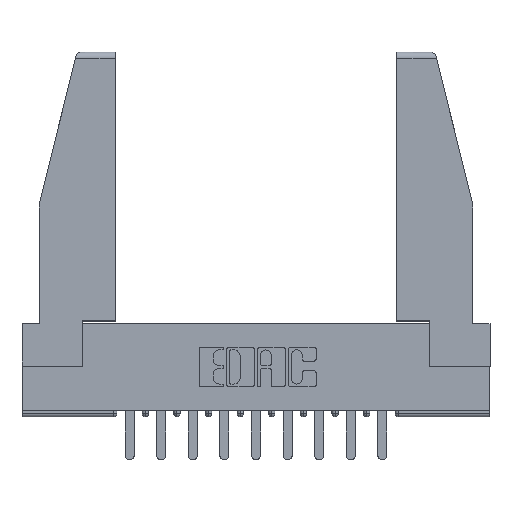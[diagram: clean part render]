
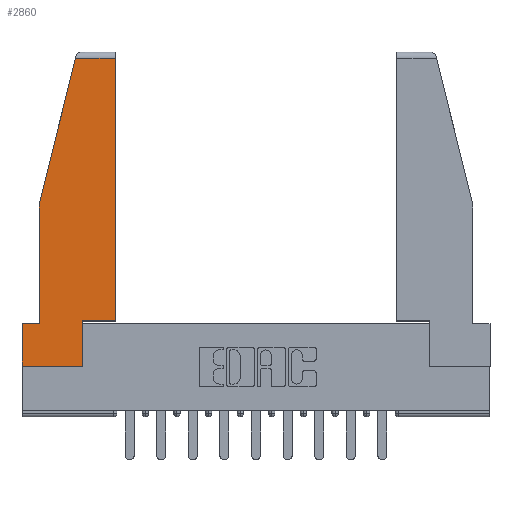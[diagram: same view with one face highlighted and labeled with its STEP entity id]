
A CAD part, top view. The second image highlights one B-rep face of the part: STEP entity #2860.
In plain terms, the highlighted planar face has unit normal (0, 0, 1).
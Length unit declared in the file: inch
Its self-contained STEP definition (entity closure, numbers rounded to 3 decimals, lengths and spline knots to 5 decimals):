
#167 = CARTESIAN_POINT ( 'NONE',  ( 0.297, 0., 0. ) ) ;
#615 = CARTESIAN_POINT ( 'NONE',  ( 0., 0., 0. ) ) ;
#668 = VECTOR ( 'NONE', #8872, 39.37008 ) ;
#1336 = ORIENTED_EDGE ( 'NONE', *, *, #2881, .T. ) ;
#1366 = VERTEX_POINT ( 'NONE', #615 ) ;
#1624 = CARTESIAN_POINT ( 'NONE',  ( 0.297, 0.223, 0. ) ) ;
#1625 = DIRECTION ( 'NONE',  ( -0.239, -0.971, 0. ) ) ;
#1884 = CARTESIAN_POINT ( 'NONE',  ( 0.461, 1.52, 0. ) ) ;
#2151 = ORIENTED_EDGE ( 'NONE', *, *, #11535, .T. ) ;
#2159 = VERTEX_POINT ( 'NONE', #7401 ) ;
#2522 = DIRECTION ( 'NONE',  ( 0., 1., 0. ) ) ;
#2757 = LINE ( 'NONE', #7891, #9374 ) ;
#2848 = VERTEX_POINT ( 'NONE', #7024 ) ;
#2860 = ADVANCED_FACE ( 'NONE', ( #3375 ), #5828, .T. ) ;
#2881 = EDGE_CURVE ( 'NONE', #3419, #1366, #15807, .T. ) ;
#2916 = VECTOR ( 'NONE', #1625, 39.37008 ) ;
#3042 = ORIENTED_EDGE ( 'NONE', *, *, #3431, .T. ) ;
#3375 = FACE_OUTER_BOUND ( 'NONE', #16056, .T. ) ;
#3419 = VERTEX_POINT ( 'NONE', #5701 ) ;
#3431 = EDGE_CURVE ( 'NONE', #12406, #16017, #2757, .T. ) ;
#3662 = DIRECTION ( 'NONE',  ( -1., 0., 0. ) ) ;
#3814 = CARTESIAN_POINT ( 'NONE',  ( 0.2636, 1.52, 0. ) ) ;
#3930 = EDGE_CURVE ( 'NONE', #10735, #2159, #7797, .T. ) ;
#4960 = CARTESIAN_POINT ( 'NONE',  ( 0.086, 0.8, 0. ) ) ;
#5069 = EDGE_CURVE ( 'NONE', #16017, #7656, #12213, .T. ) ;
#5186 = EDGE_CURVE ( 'NONE', #1366, #12444, #15535, .T. ) ;
#5538 = CARTESIAN_POINT ( 'NONE',  ( 0.271, 1.55, 0. ) ) ;
#5701 = CARTESIAN_POINT ( 'NONE',  ( 0., 0.21, 0. ) ) ;
#5828 = PLANE ( 'NONE',  #9553 ) ;
#5879 = DIRECTION ( 'NONE',  ( 1., 0., 0. ) ) ;
#5894 = LINE ( 'NONE', #167, #15965 ) ;
#6086 = EDGE_CURVE ( 'NONE', #2848, #3419, #10066, .T. ) ;
#6168 = ORIENTED_EDGE ( 'NONE', *, *, #5069, .T. ) ;
#6827 = CARTESIAN_POINT ( 'NONE',  ( 0., 0., 0. ) ) ;
#7024 = CARTESIAN_POINT ( 'NONE',  ( 0.086, 0.21, 0. ) ) ;
#7355 = ORIENTED_EDGE ( 'NONE', *, *, #5186, .T. ) ;
#7401 = CARTESIAN_POINT ( 'NONE',  ( 0.461, 0.223, 0. ) ) ;
#7409 = ORIENTED_EDGE ( 'NONE', *, *, #12938, .T. ) ;
#7519 = CARTESIAN_POINT ( 'NONE',  ( 0.297, 0.223, 0. ) ) ;
#7656 = VERTEX_POINT ( 'NONE', #10710 ) ;
#7797 = LINE ( 'NONE', #7519, #10109 ) ;
#7891 = CARTESIAN_POINT ( 'NONE',  ( 0., 1.52, 0. ) ) ;
#8137 = CARTESIAN_POINT ( 'NONE',  ( 0., 0., 0. ) ) ;
#8360 = EDGE_CURVE ( 'NONE', #2159, #12406, #10392, .T. ) ;
#8376 = ORIENTED_EDGE ( 'NONE', *, *, #3930, .T. ) ;
#8609 = ORIENTED_EDGE ( 'NONE', *, *, #6086, .T. ) ;
#8872 = DIRECTION ( 'NONE',  ( 0., 1., 0. ) ) ;
#9374 = VECTOR ( 'NONE', #15409, 39.37008 ) ;
#9481 = DIRECTION ( 'NONE',  ( 0., 0., 1. ) ) ;
#9553 = AXIS2_PLACEMENT_3D ( 'NONE', #8137, #9481, #5879 ) ;
#9976 = LINE ( 'NONE', #4960, #15448 ) ;
#10066 = LINE ( 'NONE', #13430, #11632 ) ;
#10109 = VECTOR ( 'NONE', #12290, 39.37008 ) ;
#10392 = LINE ( 'NONE', #13841, #668 ) ;
#10651 = DIRECTION ( 'NONE',  ( 1., 0., 0. ) ) ;
#10710 = CARTESIAN_POINT ( 'NONE',  ( 0.086, 0.8, 0. ) ) ;
#10735 = VERTEX_POINT ( 'NONE', #1624 ) ;
#11535 = EDGE_CURVE ( 'NONE', #7656, #2848, #9976, .T. ) ;
#11632 = VECTOR ( 'NONE', #3662, 39.37008 ) ;
#12171 = CARTESIAN_POINT ( 'NONE',  ( 0.297, 0., 0. ) ) ;
#12213 = LINE ( 'NONE', #5538, #2916 ) ;
#12290 = DIRECTION ( 'NONE',  ( 1., 0., 0. ) ) ;
#12406 = VERTEX_POINT ( 'NONE', #1884 ) ;
#12414 = VECTOR ( 'NONE', #10651, 39.37008 ) ;
#12444 = VERTEX_POINT ( 'NONE', #12171 ) ;
#12938 = EDGE_CURVE ( 'NONE', #12444, #10735, #5894, .T. ) ;
#13229 = DIRECTION ( 'NONE',  ( 0., -1., 0. ) ) ;
#13430 = CARTESIAN_POINT ( 'NONE',  ( 0., 0.21, 0. ) ) ;
#13665 = DIRECTION ( 'NONE',  ( 0., -1., 0. ) ) ;
#13841 = CARTESIAN_POINT ( 'NONE',  ( 0.461, 0.223, 0. ) ) ;
#14412 = ORIENTED_EDGE ( 'NONE', *, *, #8360, .T. ) ;
#14454 = CARTESIAN_POINT ( 'NONE',  ( 0., 0.21, 0. ) ) ;
#14821 = VECTOR ( 'NONE', #13229, 39.37008 ) ;
#15409 = DIRECTION ( 'NONE',  ( -1., 0., 0. ) ) ;
#15448 = VECTOR ( 'NONE', #13665, 39.37008 ) ;
#15535 = LINE ( 'NONE', #6827, #12414 ) ;
#15807 = LINE ( 'NONE', #14454, #14821 ) ;
#15965 = VECTOR ( 'NONE', #2522, 39.37008 ) ;
#16017 = VERTEX_POINT ( 'NONE', #3814 ) ;
#16056 = EDGE_LOOP ( 'NONE', ( #14412, #3042, #6168, #2151, #8609, #1336, #7355, #7409, #8376 ) ) ;
